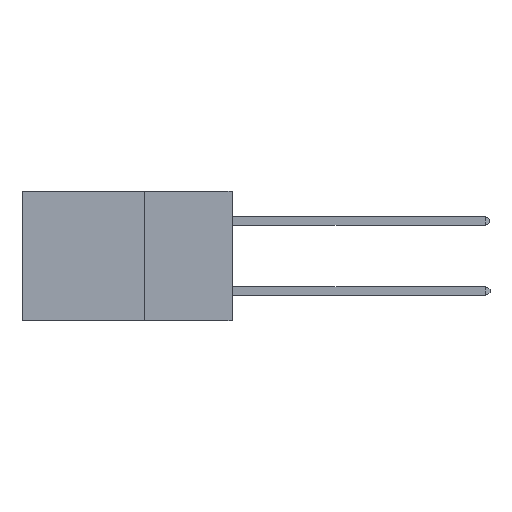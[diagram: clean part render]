
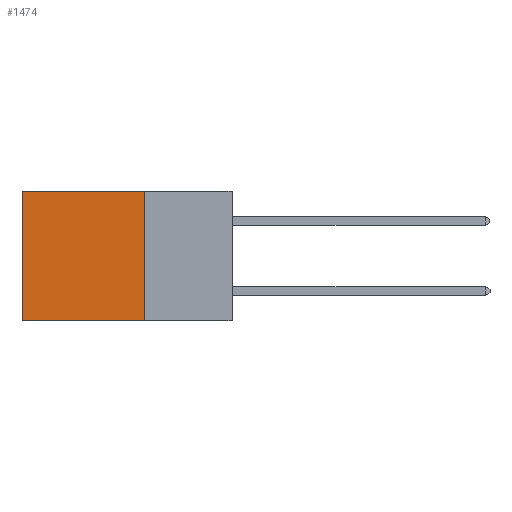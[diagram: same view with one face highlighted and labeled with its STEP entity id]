
A CAD part, left-side view. The second image highlights one B-rep face of the part: STEP entity #1474.
In plain terms, the highlighted planar face has unit normal (-1, 0, 0).
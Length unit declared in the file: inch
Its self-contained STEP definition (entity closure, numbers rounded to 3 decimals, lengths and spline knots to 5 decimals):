
#226 = VERTEX_POINT ( 'NONE', #8261 ) ;
#1136 = VERTEX_POINT ( 'NONE', #7919 ) ;
#1333 = CARTESIAN_POINT ( 'NONE',  ( 0.2875, 0.25, 0. ) ) ;
#1474 = ADVANCED_FACE ( 'NONE', ( #15790 ), #2644, .F. ) ;
#2230 = EDGE_CURVE ( 'NONE', #1136, #9123, #7030, .T. ) ;
#2644 = PLANE ( 'NONE',  #10008 ) ;
#2906 = DIRECTION ( 'NONE',  ( 0., 1., 0. ) ) ;
#3335 = CARTESIAN_POINT ( 'NONE',  ( 0.2875, 0.25, 0. ) ) ;
#3498 = VECTOR ( 'NONE', #16563, 39.37008 ) ;
#3864 = EDGE_CURVE ( 'NONE', #226, #5986, #15150, .T. ) ;
#5345 = CARTESIAN_POINT ( 'NONE',  ( 0.2875, 0.6, -0.37 ) ) ;
#5709 = DIRECTION ( 'NONE',  ( 0., 0., -1. ) ) ;
#5986 = VERTEX_POINT ( 'NONE', #18170 ) ;
#7030 = LINE ( 'NONE', #7172, #14285 ) ;
#7143 = ORIENTED_EDGE ( 'NONE', *, *, #17421, .F. ) ;
#7172 = CARTESIAN_POINT ( 'NONE',  ( 0.2875, 0.6, 0. ) ) ;
#7355 = ORIENTED_EDGE ( 'NONE', *, *, #3864, .F. ) ;
#7381 = CARTESIAN_POINT ( 'NONE',  ( 0.2875, 0.25, -0.37 ) ) ;
#7507 = ORIENTED_EDGE ( 'NONE', *, *, #15777, .T. ) ;
#7919 = CARTESIAN_POINT ( 'NONE',  ( 0.2875, 0.6, 0. ) ) ;
#8261 = CARTESIAN_POINT ( 'NONE',  ( 0.2875, 0.25, 0. ) ) ;
#8661 = DIRECTION ( 'NONE',  ( 0., 0., -1. ) ) ;
#9123 = VERTEX_POINT ( 'NONE', #5345 ) ;
#9175 = LINE ( 'NONE', #1333, #16329 ) ;
#9359 = ORIENTED_EDGE ( 'NONE', *, *, #2230, .T. ) ;
#10008 = AXIS2_PLACEMENT_3D ( 'NONE', #12964, #14418, #5709 ) ;
#10888 = LINE ( 'NONE', #7381, #17588 ) ;
#12964 = CARTESIAN_POINT ( 'NONE',  ( 0.2875, 0.25, 0. ) ) ;
#13188 = DIRECTION ( 'NONE',  ( 0., 1., 0. ) ) ;
#13504 = EDGE_LOOP ( 'NONE', ( #9359, #7143, #7355, #7507 ) ) ;
#14285 = VECTOR ( 'NONE', #8661, 39.37008 ) ;
#14418 = DIRECTION ( 'NONE',  ( 1., 0., 0. ) ) ;
#15150 = LINE ( 'NONE', #3335, #3498 ) ;
#15777 = EDGE_CURVE ( 'NONE', #226, #1136, #9175, .T. ) ;
#15790 = FACE_OUTER_BOUND ( 'NONE', #13504, .T. ) ;
#16329 = VECTOR ( 'NONE', #2906, 39.37008 ) ;
#16563 = DIRECTION ( 'NONE',  ( 0., 0., -1. ) ) ;
#17421 = EDGE_CURVE ( 'NONE', #5986, #9123, #10888, .T. ) ;
#17588 = VECTOR ( 'NONE', #13188, 39.37008 ) ;
#18170 = CARTESIAN_POINT ( 'NONE',  ( 0.2875, 0.25, -0.37 ) ) ;
